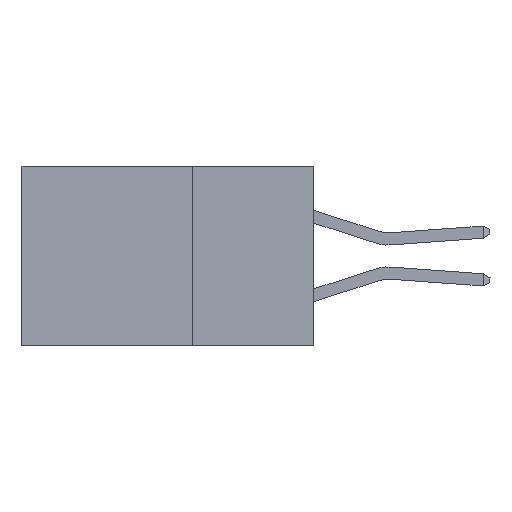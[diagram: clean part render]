
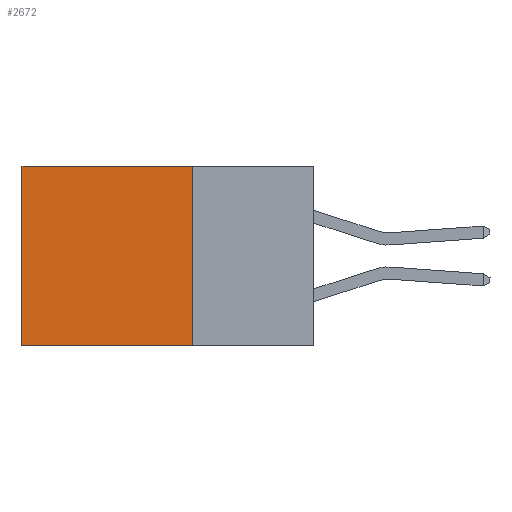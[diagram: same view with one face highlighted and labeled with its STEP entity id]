
A CAD part, left-side view. The second image highlights one B-rep face of the part: STEP entity #2672.
In plain terms, the highlighted planar face has unit normal (-1, 0, 0).
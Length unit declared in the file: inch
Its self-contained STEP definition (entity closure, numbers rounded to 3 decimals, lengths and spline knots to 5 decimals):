
#620 = CARTESIAN_POINT ( 'NONE',  ( 0.2875, 0.6, 0. ) ) ;
#644 = EDGE_CURVE ( 'NONE', #12024, #4060, #27232, .T. ) ;
#2672 = ADVANCED_FACE ( 'NONE', ( #18398 ), #25613, .F. ) ;
#4060 = VERTEX_POINT ( 'NONE', #6551 ) ;
#4940 = DIRECTION ( 'NONE',  ( 0., 0., -1. ) ) ;
#5187 = ORIENTED_EDGE ( 'NONE', *, *, #644, .T. ) ;
#6551 = CARTESIAN_POINT ( 'NONE',  ( 0.2875, 0.6, 0. ) ) ;
#6779 = ORIENTED_EDGE ( 'NONE', *, *, #30470, .T. ) ;
#8112 = VECTOR ( 'NONE', #23439, 39.37008 ) ;
#8519 = CARTESIAN_POINT ( 'NONE',  ( 0.2875, 0.25, 0. ) ) ;
#12024 = VERTEX_POINT ( 'NONE', #20059 ) ;
#12482 = ORIENTED_EDGE ( 'NONE', *, *, #35795, .F. ) ;
#13214 = AXIS2_PLACEMENT_3D ( 'NONE', #8519, #20112, #34101 ) ;
#15652 = EDGE_CURVE ( 'NONE', #29336, #31279, #18590, .T. ) ;
#16007 = CARTESIAN_POINT ( 'NONE',  ( 0.2875, 0.25, -0.37 ) ) ;
#16924 = VECTOR ( 'NONE', #27822, 39.37008 ) ;
#17368 = VECTOR ( 'NONE', #4940, 39.37008 ) ;
#18398 = FACE_OUTER_BOUND ( 'NONE', #23076, .T. ) ;
#18590 = LINE ( 'NONE', #22025, #33775 ) ;
#19645 = LINE ( 'NONE', #36891, #17368 ) ;
#20059 = CARTESIAN_POINT ( 'NONE',  ( 0.2875, 0.25, 0. ) ) ;
#20112 = DIRECTION ( 'NONE',  ( 1., 0., 0. ) ) ;
#22025 = CARTESIAN_POINT ( 'NONE',  ( 0.2875, 0.25, -0.37 ) ) ;
#23076 = EDGE_LOOP ( 'NONE', ( #6779, #36788, #12482, #5187 ) ) ;
#23439 = DIRECTION ( 'NONE',  ( 0., 0., -1. ) ) ;
#25613 = PLANE ( 'NONE',  #13214 ) ;
#26961 = CARTESIAN_POINT ( 'NONE',  ( 0.2875, 0.6, -0.37 ) ) ;
#27232 = LINE ( 'NONE', #33938, #16924 ) ;
#27822 = DIRECTION ( 'NONE',  ( 0., 1., 0. ) ) ;
#29336 = VERTEX_POINT ( 'NONE', #16007 ) ;
#30470 = EDGE_CURVE ( 'NONE', #4060, #31279, #33562, .T. ) ;
#31279 = VERTEX_POINT ( 'NONE', #26961 ) ;
#33562 = LINE ( 'NONE', #620, #8112 ) ;
#33743 = DIRECTION ( 'NONE',  ( 0., 1., 0. ) ) ;
#33775 = VECTOR ( 'NONE', #33743, 39.37008 ) ;
#33938 = CARTESIAN_POINT ( 'NONE',  ( 0.2875, 0.25, 0. ) ) ;
#34101 = DIRECTION ( 'NONE',  ( 0., 0., -1. ) ) ;
#35795 = EDGE_CURVE ( 'NONE', #12024, #29336, #19645, .T. ) ;
#36788 = ORIENTED_EDGE ( 'NONE', *, *, #15652, .F. ) ;
#36891 = CARTESIAN_POINT ( 'NONE',  ( 0.2875, 0.25, 0. ) ) ;
